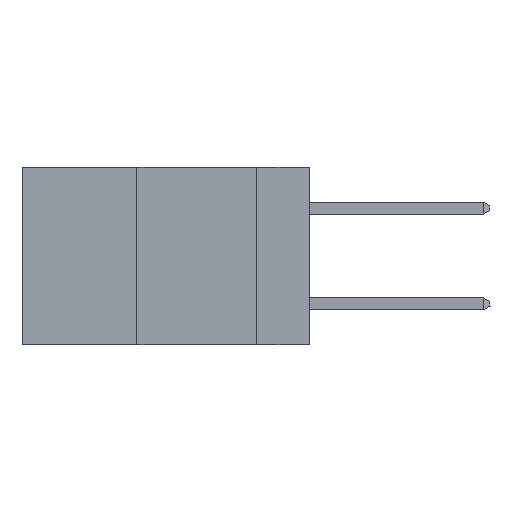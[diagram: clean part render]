
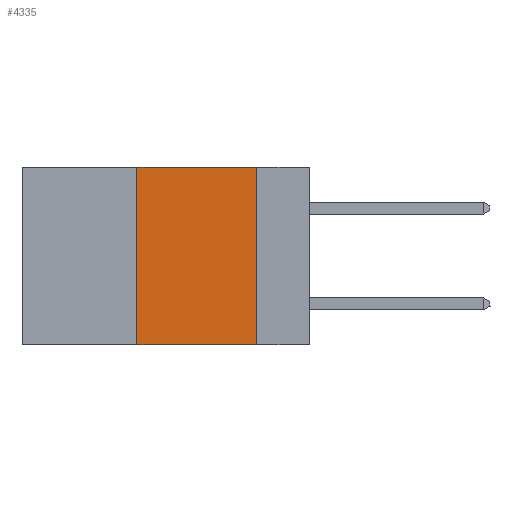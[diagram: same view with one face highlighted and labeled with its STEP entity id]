
A CAD part, left-side view. The second image highlights one B-rep face of the part: STEP entity #4335.
In plain terms, the highlighted planar face has unit normal (-1, 0, 0).
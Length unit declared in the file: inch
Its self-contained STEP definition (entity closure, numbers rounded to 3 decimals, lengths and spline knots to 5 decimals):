
#416 = CARTESIAN_POINT ( 'NONE',  ( 0., 0.11, -0.37 ) ) ;
#1249 = VERTEX_POINT ( 'NONE', #10735 ) ;
#1314 = CARTESIAN_POINT ( 'NONE',  ( 0., 0.6, 0. ) ) ;
#2484 = VECTOR ( 'NONE', #5988, 39.37008 ) ;
#2582 = EDGE_CURVE ( 'NONE', #16989, #6623, #16287, .T. ) ;
#3486 = LINE ( 'NONE', #3508, #13056 ) ;
#3508 = CARTESIAN_POINT ( 'NONE',  ( 0., 0.6, -0.37 ) ) ;
#3561 = CARTESIAN_POINT ( 'NONE',  ( 0., 0.11, 0. ) ) ;
#3863 = ORIENTED_EDGE ( 'NONE', *, *, #13010, .F. ) ;
#4003 = DIRECTION ( 'NONE',  ( 1., 0., 0. ) ) ;
#4289 = CARTESIAN_POINT ( 'NONE',  ( 0., 0.36, 0. ) ) ;
#4320 = VECTOR ( 'NONE', #10203, 39.37008 ) ;
#4335 = ADVANCED_FACE ( 'NONE', ( #10767 ), #5283, .F. ) ;
#4836 = EDGE_CURVE ( 'NONE', #1249, #16989, #17296, .T. ) ;
#5028 = DIRECTION ( 'NONE',  ( 0., -1., 0. ) ) ;
#5283 = PLANE ( 'NONE',  #11882 ) ;
#5405 = ORIENTED_EDGE ( 'NONE', *, *, #7764, .T. ) ;
#5988 = DIRECTION ( 'NONE',  ( 0., 0., 1. ) ) ;
#6059 = CARTESIAN_POINT ( 'NONE',  ( 0., 0.36, 0. ) ) ;
#6623 = VERTEX_POINT ( 'NONE', #3561 ) ;
#6712 = VERTEX_POINT ( 'NONE', #416 ) ;
#7085 = DIRECTION ( 'NONE',  ( 0., 0., -1. ) ) ;
#7764 = EDGE_CURVE ( 'NONE', #1249, #6712, #3486, .T. ) ;
#7890 = ORIENTED_EDGE ( 'NONE', *, *, #4836, .F. ) ;
#10203 = DIRECTION ( 'NONE',  ( 0., -1., 0. ) ) ;
#10638 = EDGE_LOOP ( 'NONE', ( #3863, #14143, #7890, #5405 ) ) ;
#10735 = CARTESIAN_POINT ( 'NONE',  ( 0., 0.36, -0.37 ) ) ;
#10767 = FACE_OUTER_BOUND ( 'NONE', #10638, .T. ) ;
#11844 = LINE ( 'NONE', #14011, #17736 ) ;
#11882 = AXIS2_PLACEMENT_3D ( 'NONE', #1314, #4003, #13731 ) ;
#13010 = EDGE_CURVE ( 'NONE', #6623, #6712, #11844, .T. ) ;
#13056 = VECTOR ( 'NONE', #5028, 39.37008 ) ;
#13731 = DIRECTION ( 'NONE',  ( 0., 0., -1. ) ) ;
#14011 = CARTESIAN_POINT ( 'NONE',  ( 0., 0.11, 0. ) ) ;
#14143 = ORIENTED_EDGE ( 'NONE', *, *, #2582, .F. ) ;
#14490 = CARTESIAN_POINT ( 'NONE',  ( 0., 0.6, 0. ) ) ;
#16287 = LINE ( 'NONE', #14490, #4320 ) ;
#16989 = VERTEX_POINT ( 'NONE', #6059 ) ;
#17296 = LINE ( 'NONE', #4289, #2484 ) ;
#17736 = VECTOR ( 'NONE', #7085, 39.37008 ) ;
